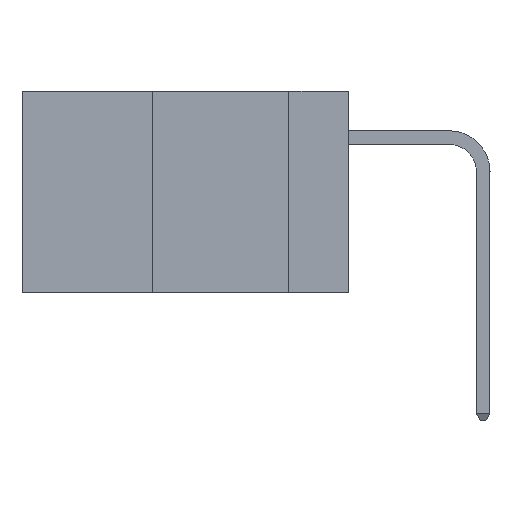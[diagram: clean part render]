
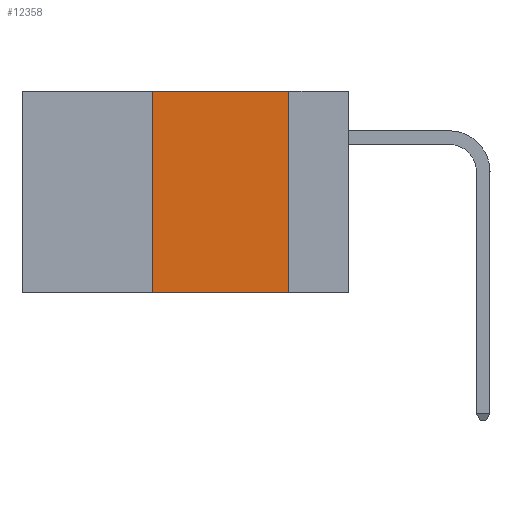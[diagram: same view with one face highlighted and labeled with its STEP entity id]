
A CAD part, left-side view. The second image highlights one B-rep face of the part: STEP entity #12358.
In plain terms, the highlighted planar face has unit normal (-1, 0, 0).
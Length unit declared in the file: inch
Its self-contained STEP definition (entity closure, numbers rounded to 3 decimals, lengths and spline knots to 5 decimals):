
#481 = DIRECTION ( 'NONE',  ( 1., 0., 0. ) ) ;
#500 = EDGE_LOOP ( 'NONE', ( #36680, #2476, #22127, #9504 ) ) ;
#700 = CARTESIAN_POINT ( 'NONE',  ( 0., 0.36, -0.37 ) ) ;
#2476 = ORIENTED_EDGE ( 'NONE', *, *, #33399, .F. ) ;
#3671 = DIRECTION ( 'NONE',  ( 0., 0., 1. ) ) ;
#4382 = CARTESIAN_POINT ( 'NONE',  ( 0., 0.6, -0.37 ) ) ;
#6734 = VECTOR ( 'NONE', #3671, 39.37008 ) ;
#7624 = VERTEX_POINT ( 'NONE', #700 ) ;
#8930 = VECTOR ( 'NONE', #34151, 39.37008 ) ;
#9093 = EDGE_CURVE ( 'NONE', #7624, #23142, #32441, .T. ) ;
#9110 = VERTEX_POINT ( 'NONE', #21768 ) ;
#9504 = ORIENTED_EDGE ( 'NONE', *, *, #9093, .T. ) ;
#12358 = ADVANCED_FACE ( 'NONE', ( #28957 ), #35411, .F. ) ;
#12914 = CARTESIAN_POINT ( 'NONE',  ( 0., 0.36, 0. ) ) ;
#15324 = CARTESIAN_POINT ( 'NONE',  ( 0., 0.36, 0. ) ) ;
#15363 = LINE ( 'NONE', #15324, #6734 ) ;
#16841 = DIRECTION ( 'NONE',  ( 0., 0., -1. ) ) ;
#17875 = VECTOR ( 'NONE', #24669, 39.37008 ) ;
#18014 = CARTESIAN_POINT ( 'NONE',  ( 0., 0.6, 0. ) ) ;
#18245 = AXIS2_PLACEMENT_3D ( 'NONE', #18014, #481, #20897 ) ;
#20627 = CARTESIAN_POINT ( 'NONE',  ( 0., 0.11, -0.37 ) ) ;
#20897 = DIRECTION ( 'NONE',  ( 0., 0., -1. ) ) ;
#21768 = CARTESIAN_POINT ( 'NONE',  ( 0., 0.11, 0. ) ) ;
#22127 = ORIENTED_EDGE ( 'NONE', *, *, #27269, .F. ) ;
#23142 = VERTEX_POINT ( 'NONE', #20627 ) ;
#24669 = DIRECTION ( 'NONE',  ( 0., -1., 0. ) ) ;
#27269 = EDGE_CURVE ( 'NONE', #7624, #29245, #15363, .T. ) ;
#28957 = FACE_OUTER_BOUND ( 'NONE', #500, .T. ) ;
#29245 = VERTEX_POINT ( 'NONE', #12914 ) ;
#29964 = EDGE_CURVE ( 'NONE', #9110, #23142, #31546, .T. ) ;
#30645 = VECTOR ( 'NONE', #16841, 39.37008 ) ;
#31259 = CARTESIAN_POINT ( 'NONE',  ( 0., 0.6, 0. ) ) ;
#31336 = CARTESIAN_POINT ( 'NONE',  ( 0., 0.11, 0. ) ) ;
#31546 = LINE ( 'NONE', #31336, #30645 ) ;
#32082 = LINE ( 'NONE', #31259, #8930 ) ;
#32441 = LINE ( 'NONE', #4382, #17875 ) ;
#33399 = EDGE_CURVE ( 'NONE', #29245, #9110, #32082, .T. ) ;
#34151 = DIRECTION ( 'NONE',  ( 0., -1., 0. ) ) ;
#35411 = PLANE ( 'NONE',  #18245 ) ;
#36680 = ORIENTED_EDGE ( 'NONE', *, *, #29964, .F. ) ;
